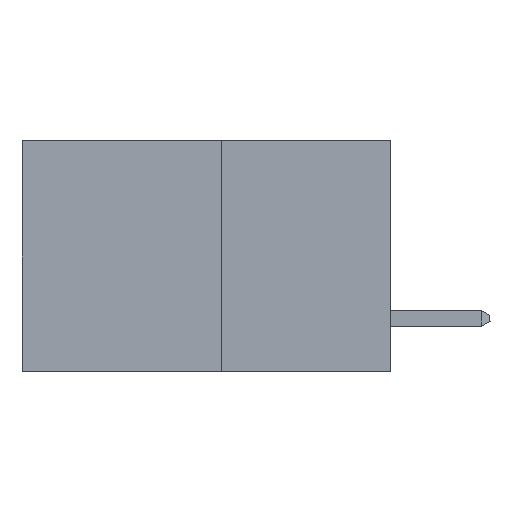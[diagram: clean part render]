
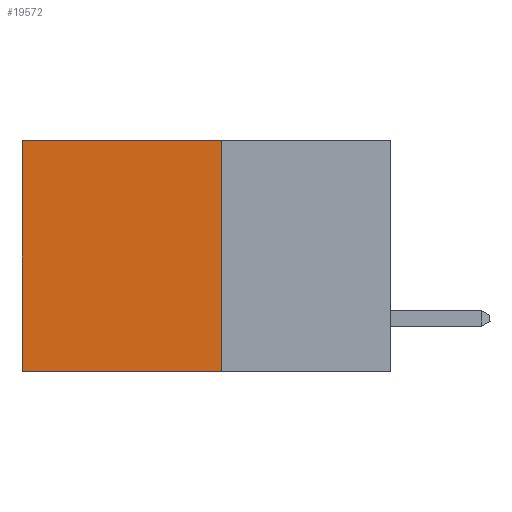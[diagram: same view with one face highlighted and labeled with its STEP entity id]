
A CAD part, left-side view. The second image highlights one B-rep face of the part: STEP entity #19572.
In plain terms, the highlighted planar face has unit normal (-1, 0, 0).
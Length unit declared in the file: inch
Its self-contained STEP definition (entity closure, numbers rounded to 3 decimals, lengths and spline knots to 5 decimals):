
#694 = DIRECTION ( 'NONE',  ( 0., 0., -1. ) ) ;
#1137 = VECTOR ( 'NONE', #20435, 39.37008 ) ;
#1458 = LINE ( 'NONE', #20695, #14884 ) ;
#2350 = ORIENTED_EDGE ( 'NONE', *, *, #14916, .T. ) ;
#5698 = DIRECTION ( 'NONE',  ( 0., 0., -1. ) ) ;
#5700 = VECTOR ( 'NONE', #16206, 39.37008 ) ;
#6145 = CARTESIAN_POINT ( 'NONE',  ( 0.277, 0.27, -0.37 ) ) ;
#6182 = VERTEX_POINT ( 'NONE', #23652 ) ;
#8247 = DIRECTION ( 'NONE',  ( 0., 1., 0. ) ) ;
#8321 = PLANE ( 'NONE',  #21572 ) ;
#8529 = EDGE_CURVE ( 'NONE', #6182, #11853, #21988, .T. ) ;
#9495 = VECTOR ( 'NONE', #8247, 39.37008 ) ;
#9525 = LINE ( 'NONE', #17935, #1137 ) ;
#9786 = ORIENTED_EDGE ( 'NONE', *, *, #17113, .F. ) ;
#10862 = CARTESIAN_POINT ( 'NONE',  ( 0.277, 0.27, -0.37 ) ) ;
#11853 = VERTEX_POINT ( 'NONE', #16229 ) ;
#11961 = ORIENTED_EDGE ( 'NONE', *, *, #12811, .T. ) ;
#12390 = LINE ( 'NONE', #6145, #5700 ) ;
#12771 = ORIENTED_EDGE ( 'NONE', *, *, #8529, .F. ) ;
#12811 = EDGE_CURVE ( 'NONE', #31154, #28008, #9525, .T. ) ;
#13394 = CARTESIAN_POINT ( 'NONE',  ( 0.277, 0.59, 0. ) ) ;
#14884 = VECTOR ( 'NONE', #5698, 39.37008 ) ;
#14916 = EDGE_CURVE ( 'NONE', #28008, #11853, #1458, .T. ) ;
#15842 = DIRECTION ( 'NONE',  ( 1., 0., 0. ) ) ;
#16206 = DIRECTION ( 'NONE',  ( 0., 0., -1. ) ) ;
#16229 = CARTESIAN_POINT ( 'NONE',  ( 0.277, 0.59, -0.37 ) ) ;
#16938 = FACE_OUTER_BOUND ( 'NONE', #16971, .T. ) ;
#16971 = EDGE_LOOP ( 'NONE', ( #2350, #12771, #9786, #11961 ) ) ;
#17113 = EDGE_CURVE ( 'NONE', #31154, #6182, #12390, .T. ) ;
#17935 = CARTESIAN_POINT ( 'NONE',  ( 0.277, 0.27, 0. ) ) ;
#19572 = ADVANCED_FACE ( 'NONE', ( #16938 ), #8321, .F. ) ;
#20435 = DIRECTION ( 'NONE',  ( 0., 1., 0. ) ) ;
#20695 = CARTESIAN_POINT ( 'NONE',  ( 0.277, 0.59, -0.37 ) ) ;
#21572 = AXIS2_PLACEMENT_3D ( 'NONE', #30771, #15842, #694 ) ;
#21988 = LINE ( 'NONE', #10862, #9495 ) ;
#23652 = CARTESIAN_POINT ( 'NONE',  ( 0.277, 0.27, -0.37 ) ) ;
#28008 = VERTEX_POINT ( 'NONE', #13394 ) ;
#30542 = CARTESIAN_POINT ( 'NONE',  ( 0.277, 0.27, 0. ) ) ;
#30771 = CARTESIAN_POINT ( 'NONE',  ( 0.277, 0.27, -0.37 ) ) ;
#31154 = VERTEX_POINT ( 'NONE', #30542 ) ;
